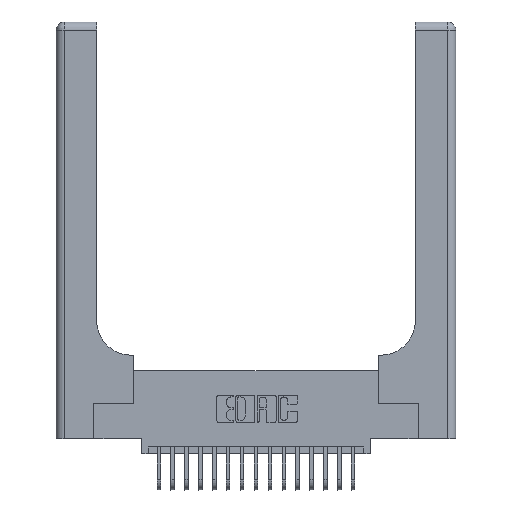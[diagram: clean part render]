
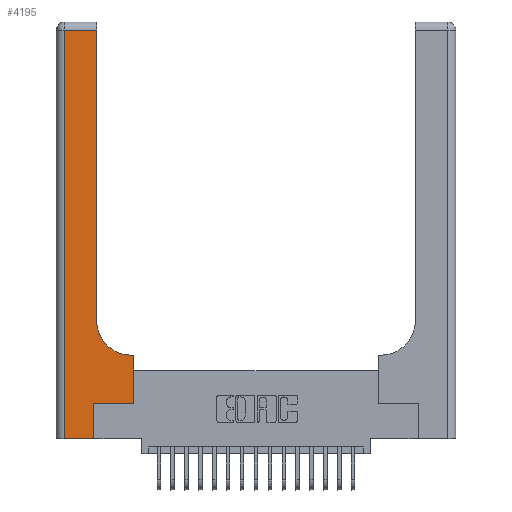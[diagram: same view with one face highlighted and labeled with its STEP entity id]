
A CAD part, top view. The second image highlights one B-rep face of the part: STEP entity #4195.
In plain terms, the highlighted planar face has unit normal (0, 0, 1).
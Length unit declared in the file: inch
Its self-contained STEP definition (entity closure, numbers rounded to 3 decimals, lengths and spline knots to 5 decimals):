
#262 = DIRECTION ( 'NONE',  ( 0., 1., 0. ) ) ;
#728 = DIRECTION ( 'NONE',  ( -1., 0., 0. ) ) ;
#759 = EDGE_CURVE ( 'NONE', #19703, #19818, #10569, .T. ) ;
#764 = EDGE_CURVE ( 'NONE', #12415, #19703, #14627, .T. ) ;
#998 = LINE ( 'NONE', #17653, #6910 ) ;
#1383 = CARTESIAN_POINT ( 'NONE',  ( 0., 2.94, 0.37 ) ) ;
#1602 = LINE ( 'NONE', #1383, #13482 ) ;
#2028 = DIRECTION ( 'NONE',  ( -1., 0., 0. ) ) ;
#2658 = ORIENTED_EDGE ( 'NONE', *, *, #764, .T. ) ;
#3369 = VECTOR ( 'NONE', #4405, 39.37008 ) ;
#3578 = DIRECTION ( 'NONE',  ( 0., 1., 0. ) ) ;
#3676 = VERTEX_POINT ( 'NONE', #7499 ) ;
#3888 = EDGE_CURVE ( 'NONE', #3676, #7942, #1602, .T. ) ;
#3985 = DIRECTION ( 'NONE',  ( 1., 0., 0. ) ) ;
#4195 = ADVANCED_FACE ( 'NONE', ( #9379 ), #17639, .F. ) ;
#4255 = VECTOR ( 'NONE', #20220, 39.37008 ) ;
#4330 = CARTESIAN_POINT ( 'NONE',  ( 0.06, 3., 0.37 ) ) ;
#4405 = DIRECTION ( 'NONE',  ( 0., -1., 0. ) ) ;
#4422 = ORIENTED_EDGE ( 'NONE', *, *, #11331, .T. ) ;
#4461 = AXIS2_PLACEMENT_3D ( 'NONE', #19336, #14244, #10749 ) ;
#4735 = LINE ( 'NONE', #8428, #6871 ) ;
#4928 = VECTOR ( 'NONE', #3985, 39.37008 ) ;
#5240 = EDGE_LOOP ( 'NONE', ( #6715, #19096, #11870, #11772, #4422, #2658, #19184, #17927, #11668 ) ) ;
#5596 = EDGE_CURVE ( 'NONE', #19818, #16971, #18021, .T. ) ;
#6223 = DIRECTION ( 'NONE',  ( 1., 0., 0. ) ) ;
#6715 = ORIENTED_EDGE ( 'NONE', *, *, #11302, .T. ) ;
#6871 = VECTOR ( 'NONE', #22128, 39.37008 ) ;
#6910 = VECTOR ( 'NONE', #6223, 39.37008 ) ;
#7190 = CARTESIAN_POINT ( 'NONE',  ( 0.5585, 0.25, 0.37 ) ) ;
#7434 = CARTESIAN_POINT ( 'NONE',  ( 0.269, 0.25, 0.37 ) ) ;
#7499 = CARTESIAN_POINT ( 'NONE',  ( 0.2915, 2.94, 0.37 ) ) ;
#7870 = AXIS2_PLACEMENT_3D ( 'NONE', #12365, #15986, #2028 ) ;
#7942 = VERTEX_POINT ( 'NONE', #9183 ) ;
#8428 = CARTESIAN_POINT ( 'NONE',  ( 0.269, 0., 0.37 ) ) ;
#8829 = CARTESIAN_POINT ( 'NONE',  ( 0.5585, 0.6, 0.37 ) ) ;
#9140 = CARTESIAN_POINT ( 'NONE',  ( 0.269, 0.25, 0.37 ) ) ;
#9183 = CARTESIAN_POINT ( 'NONE',  ( 0.06, 2.94, 0.37 ) ) ;
#9379 = FACE_OUTER_BOUND ( 'NONE', #5240, .T. ) ;
#10428 = EDGE_CURVE ( 'NONE', #18853, #18143, #998, .T. ) ;
#10569 = LINE ( 'NONE', #7190, #21186 ) ;
#10749 = DIRECTION ( 'NONE',  ( 1., 0., 0. ) ) ;
#11228 = CIRCLE ( 'NONE', #4461, 0.25 ) ;
#11302 = EDGE_CURVE ( 'NONE', #20429, #3676, #20194, .T. ) ;
#11331 = EDGE_CURVE ( 'NONE', #18143, #12415, #4735, .T. ) ;
#11668 = ORIENTED_EDGE ( 'NONE', *, *, #21083, .T. ) ;
#11772 = ORIENTED_EDGE ( 'NONE', *, *, #10428, .T. ) ;
#11870 = ORIENTED_EDGE ( 'NONE', *, *, #15487, .T. ) ;
#12164 = CARTESIAN_POINT ( 'NONE',  ( 0.5585, 0.25, 0.37 ) ) ;
#12165 = CARTESIAN_POINT ( 'NONE',  ( 0.2915, 3., 0.37 ) ) ;
#12365 = CARTESIAN_POINT ( 'NONE',  ( 0., 3., 0.37 ) ) ;
#12415 = VERTEX_POINT ( 'NONE', #7434 ) ;
#12851 = CARTESIAN_POINT ( 'NONE',  ( 0.269, 0., 0.37 ) ) ;
#13482 = VECTOR ( 'NONE', #728, 39.37008 ) ;
#14244 = DIRECTION ( 'NONE',  ( 0., 0., -1. ) ) ;
#14615 = CARTESIAN_POINT ( 'NONE',  ( 0.06, 0., 0.37 ) ) ;
#14627 = LINE ( 'NONE', #9140, #4928 ) ;
#15487 = EDGE_CURVE ( 'NONE', #7942, #18853, #19865, .T. ) ;
#15561 = VECTOR ( 'NONE', #3578, 39.37008 ) ;
#15716 = CARTESIAN_POINT ( 'NONE',  ( 0.2915, 0.85, 0.37 ) ) ;
#15986 = DIRECTION ( 'NONE',  ( 0., 0., -1. ) ) ;
#16971 = VERTEX_POINT ( 'NONE', #20517 ) ;
#17639 = PLANE ( 'NONE',  #7870 ) ;
#17653 = CARTESIAN_POINT ( 'NONE',  ( 0., 0., 0.37 ) ) ;
#17927 = ORIENTED_EDGE ( 'NONE', *, *, #5596, .T. ) ;
#18021 = LINE ( 'NONE', #22228, #4255 ) ;
#18143 = VERTEX_POINT ( 'NONE', #12851 ) ;
#18853 = VERTEX_POINT ( 'NONE', #14615 ) ;
#19096 = ORIENTED_EDGE ( 'NONE', *, *, #3888, .T. ) ;
#19184 = ORIENTED_EDGE ( 'NONE', *, *, #759, .T. ) ;
#19336 = CARTESIAN_POINT ( 'NONE',  ( 0.5415, 0.85, 0.37 ) ) ;
#19703 = VERTEX_POINT ( 'NONE', #12164 ) ;
#19818 = VERTEX_POINT ( 'NONE', #8829 ) ;
#19865 = LINE ( 'NONE', #4330, #3369 ) ;
#20194 = LINE ( 'NONE', #12165, #15561 ) ;
#20220 = DIRECTION ( 'NONE',  ( -1., 0., 0. ) ) ;
#20429 = VERTEX_POINT ( 'NONE', #15716 ) ;
#20517 = CARTESIAN_POINT ( 'NONE',  ( 0.5415, 0.6, 0.37 ) ) ;
#21083 = EDGE_CURVE ( 'NONE', #16971, #20429, #11228, .T. ) ;
#21186 = VECTOR ( 'NONE', #262, 39.37008 ) ;
#22128 = DIRECTION ( 'NONE',  ( 0., 1., 0. ) ) ;
#22228 = CARTESIAN_POINT ( 'NONE',  ( 0.2915, 0.6, 0.37 ) ) ;
